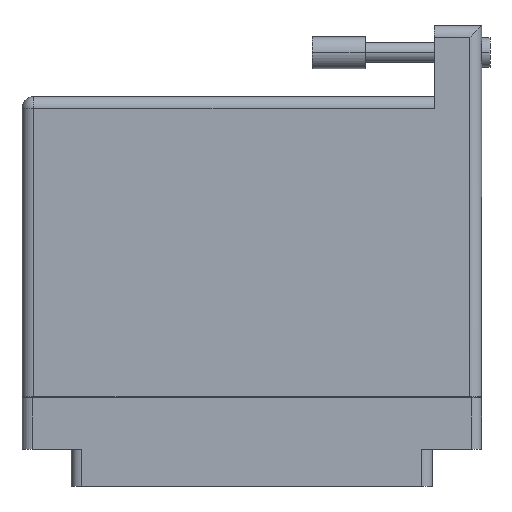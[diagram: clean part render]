
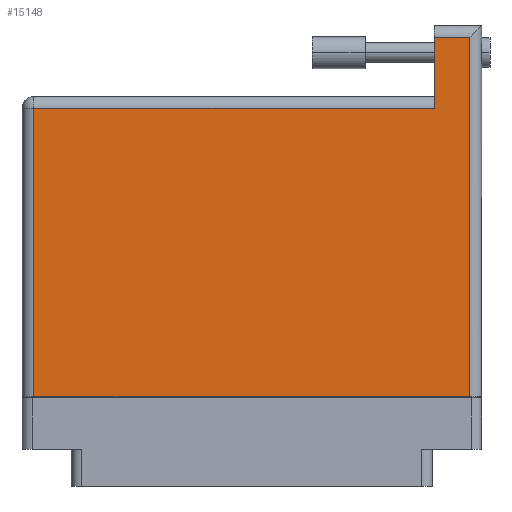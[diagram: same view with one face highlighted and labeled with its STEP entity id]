
A CAD part, front view. The second image highlights one B-rep face of the part: STEP entity #15148.
In plain terms, the highlighted face is planar.
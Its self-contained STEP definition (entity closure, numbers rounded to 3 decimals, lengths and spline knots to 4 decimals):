
#121 = EDGE_CURVE ( 'NONE', #43613, #36597, #60059, .T. ) ;
#191 = ORIENTED_EDGE ( 'NONE', *, *, #40403, .T. ) ;
#2158 = CARTESIAN_POINT ( 'NONE',  ( -1.359, 1.605, 0.617 ) ) ;
#7294 = DIRECTION ( 'NONE',  ( -1., 0., 0. ) ) ;
#7474 = CARTESIAN_POINT ( 'NONE',  ( -1.289, -0.1, 0.617 ) ) ;
#8600 = EDGE_CURVE ( 'NONE', #35787, #35680, #39535, .T. ) ;
#9530 = PLANE ( 'NONE',  #13435 ) ;
#10959 = VECTOR ( 'NONE', #7294, 39.3701 ) ;
#11030 = CARTESIAN_POINT ( 'NONE',  ( -1.289, -0.1, 0.617 ) ) ;
#13435 = AXIS2_PLACEMENT_3D ( 'NONE', #34660, #14113, #44500 ) ;
#14113 = DIRECTION ( 'NONE',  ( 0., 0., -1. ) ) ;
#15148 = ADVANCED_FACE ( 'NONE', ( #48450 ), #9530, .F. ) ;
#17274 = ORIENTED_EDGE ( 'NONE', *, *, #121, .T. ) ;
#18508 = DIRECTION ( 'NONE',  ( -1., 0., 0. ) ) ;
#19479 = CARTESIAN_POINT ( 'NONE',  ( 1.079, 2.095, 0.617 ) ) ;
#19651 = VECTOR ( 'NONE', #61602, 39.3701 ) ;
#21829 = ORIENTED_EDGE ( 'NONE', *, *, #28109, .T. ) ;
#24434 = ORIENTED_EDGE ( 'NONE', *, *, #8600, .T. ) ;
#26862 = CARTESIAN_POINT ( 'NONE',  ( 1.289, 2.095, 0.617 ) ) ;
#27253 = VECTOR ( 'NONE', #18508, 39.3701 ) ;
#28109 = EDGE_CURVE ( 'NONE', #51560, #43613, #64421, .T. ) ;
#31766 = VERTEX_POINT ( 'NONE', #36344 ) ;
#33078 = CARTESIAN_POINT ( 'NONE',  ( -1.359, -0.1, 0.617 ) ) ;
#33618 = ORIENTED_EDGE ( 'NONE', *, *, #53886, .T. ) ;
#34645 = EDGE_CURVE ( 'NONE', #35680, #31766, #53708, .T. ) ;
#34660 = CARTESIAN_POINT ( 'NONE',  ( -1.359, 1.675, 0.617 ) ) ;
#35680 = VERTEX_POINT ( 'NONE', #44657 ) ;
#35787 = VERTEX_POINT ( 'NONE', #52524 ) ;
#36344 = CARTESIAN_POINT ( 'NONE',  ( -1.289, 1.605, 0.617 ) ) ;
#36597 = VERTEX_POINT ( 'NONE', #61223 ) ;
#36965 = LINE ( 'NONE', #11030, #40912 ) ;
#37475 = EDGE_LOOP ( 'NONE', ( #52778, #191, #21829, #17274, #33618, #24434 ) ) ;
#38780 = VECTOR ( 'NONE', #47248, 39.3701 ) ;
#39535 = LINE ( 'NONE', #19479, #41139 ) ;
#40403 = EDGE_CURVE ( 'NONE', #31766, #51560, #36965, .T. ) ;
#40912 = VECTOR ( 'NONE', #41183, 39.3701 ) ;
#41139 = VECTOR ( 'NONE', #44976, 39.3701 ) ;
#41183 = DIRECTION ( 'NONE',  ( 0., -1., 0. ) ) ;
#43613 = VERTEX_POINT ( 'NONE', #61806 ) ;
#44500 = DIRECTION ( 'NONE',  ( -1., 0., 0. ) ) ;
#44657 = CARTESIAN_POINT ( 'NONE',  ( 1.079, 1.605, 0.617 ) ) ;
#44976 = DIRECTION ( 'NONE',  ( 0., -1., 0. ) ) ;
#47248 = DIRECTION ( 'NONE',  ( 1., 0., 0. ) ) ;
#48450 = FACE_OUTER_BOUND ( 'NONE', #37475, .T. ) ;
#50722 = LINE ( 'NONE', #57998, #10959 ) ;
#51560 = VERTEX_POINT ( 'NONE', #7474 ) ;
#52524 = CARTESIAN_POINT ( 'NONE',  ( 1.079, 2.025, 0.617 ) ) ;
#52778 = ORIENTED_EDGE ( 'NONE', *, *, #34645, .T. ) ;
#53708 = LINE ( 'NONE', #2158, #27253 ) ;
#53886 = EDGE_CURVE ( 'NONE', #36597, #35787, #50722, .T. ) ;
#57998 = CARTESIAN_POINT ( 'NONE',  ( -1.359, 2.025, 0.617 ) ) ;
#60059 = LINE ( 'NONE', #26862, #19651 ) ;
#61223 = CARTESIAN_POINT ( 'NONE',  ( 1.289, 2.025, 0.617 ) ) ;
#61602 = DIRECTION ( 'NONE',  ( 0., 1., 0. ) ) ;
#61806 = CARTESIAN_POINT ( 'NONE',  ( 1.289, -0.1, 0.617 ) ) ;
#64421 = LINE ( 'NONE', #33078, #38780 ) ;
